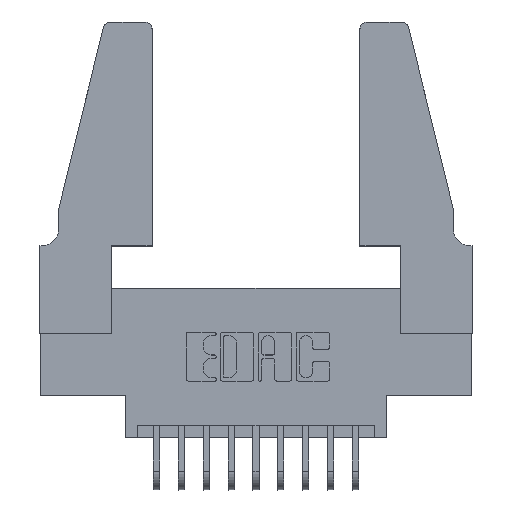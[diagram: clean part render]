
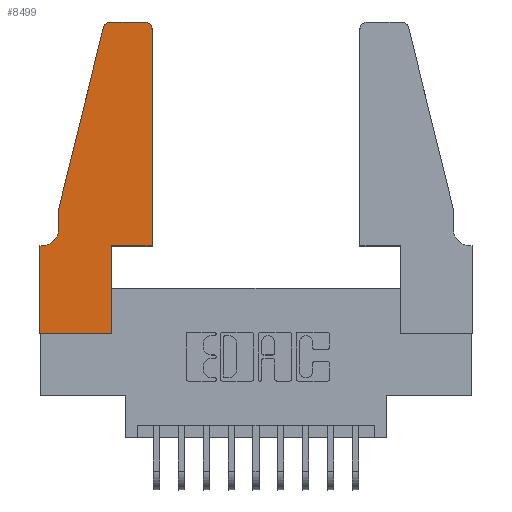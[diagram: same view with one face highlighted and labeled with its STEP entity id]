
A CAD part, top view. The second image highlights one B-rep face of the part: STEP entity #8499.
In plain terms, the highlighted planar face has unit normal (0, 0, 1).
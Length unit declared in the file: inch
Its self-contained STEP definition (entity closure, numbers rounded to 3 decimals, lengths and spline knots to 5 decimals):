
#67 = DIRECTION ( 'NONE',  ( 0., -1., 0. ) ) ;
#287 = ORIENTED_EDGE ( 'NONE', *, *, #6529, .T. ) ;
#686 = CARTESIAN_POINT ( 'NONE',  ( 0.0755, 0.35, 0.37 ) ) ;
#770 = DIRECTION ( 'NONE',  ( 1., 0., 0. ) ) ;
#864 = CIRCLE ( 'NONE', #10006, 0.03 ) ;
#869 = VERTEX_POINT ( 'NONE', #8610 ) ;
#890 = DIRECTION ( 'NONE',  ( -0.239, -0.971, 0. ) ) ;
#1489 = AXIS2_PLACEMENT_3D ( 'NONE', #1945, #5606, #13711 ) ;
#1795 = ORIENTED_EDGE ( 'NONE', *, *, #4038, .T. ) ;
#1843 = CARTESIAN_POINT ( 'NONE',  ( 0.0755, 0.42, 0.37 ) ) ;
#1945 = CARTESIAN_POINT ( 'NONE',  ( 0., 0.35, 0.37 ) ) ;
#1946 = VECTOR ( 'NONE', #9826, 39.37008 ) ;
#2008 = CARTESIAN_POINT ( 'NONE',  ( 0.4505, 0.35, 0.37 ) ) ;
#2247 = CARTESIAN_POINT ( 'NONE',  ( 0.284, 1.25, 0.37 ) ) ;
#2280 = VECTOR ( 'NONE', #3668, 39.37008 ) ;
#2497 = VECTOR ( 'NONE', #770, 39.37008 ) ;
#2616 = ORIENTED_EDGE ( 'NONE', *, *, #10988, .T. ) ;
#2724 = LINE ( 'NONE', #686, #8620 ) ;
#2897 = VERTEX_POINT ( 'NONE', #1843 ) ;
#3255 = CARTESIAN_POINT ( 'NONE',  ( 0.25487, 1.22718, 0.37 ) ) ;
#3314 = EDGE_CURVE ( 'NONE', #12942, #4967, #11859, .T. ) ;
#3324 = VERTEX_POINT ( 'NONE', #8568 ) ;
#3341 = DIRECTION ( 'NONE',  ( 1., 0., 0. ) ) ;
#3425 = ORIENTED_EDGE ( 'NONE', *, *, #8893, .T. ) ;
#3594 = VERTEX_POINT ( 'NONE', #8974 ) ;
#3668 = DIRECTION ( 'NONE',  ( 0., -1., 0. ) ) ;
#4038 = EDGE_CURVE ( 'NONE', #14106, #3324, #4765, .T. ) ;
#4055 = VECTOR ( 'NONE', #3341, 39.37008 ) ;
#4428 = CARTESIAN_POINT ( 'NONE',  ( 0.2605, 1.25, 0.37 ) ) ;
#4483 = FACE_OUTER_BOUND ( 'NONE', #13383, .T. ) ;
#4545 = CARTESIAN_POINT ( 'NONE',  ( 0., 0., 0.37 ) ) ;
#4765 = LINE ( 'NONE', #8649, #10584 ) ;
#4893 = VERTEX_POINT ( 'NONE', #3255 ) ;
#4896 = ORIENTED_EDGE ( 'NONE', *, *, #7492, .T. ) ;
#4967 = VERTEX_POINT ( 'NONE', #13349 ) ;
#5037 = DIRECTION ( 'NONE',  ( 0., 0., -1. ) ) ;
#5199 = LINE ( 'NONE', #14412, #1946 ) ;
#5317 = CARTESIAN_POINT ( 'NONE',  ( 0.284, 1.22, 0.37 ) ) ;
#5606 = DIRECTION ( 'NONE',  ( 0., 0., 1. ) ) ;
#6224 = DIRECTION ( 'NONE',  ( 0., 0., 1. ) ) ;
#6474 = DIRECTION ( 'NONE',  ( 1., 0., 0. ) ) ;
#6529 = EDGE_CURVE ( 'NONE', #2897, #3594, #13419, .T. ) ;
#6693 = LINE ( 'NONE', #4428, #9792 ) ;
#7492 = EDGE_CURVE ( 'NONE', #11521, #12942, #12670, .T. ) ;
#7604 = AXIS2_PLACEMENT_3D ( 'NONE', #11986, #5037, #13156 ) ;
#7667 = LINE ( 'NONE', #8152, #13856 ) ;
#7758 = CARTESIAN_POINT ( 'NONE',  ( 0.4505, 0.35, 0.37 ) ) ;
#7877 = LINE ( 'NONE', #9168, #4055 ) ;
#7952 = DIRECTION ( 'NONE',  ( 0., 1., 0. ) ) ;
#7994 = CARTESIAN_POINT ( 'NONE',  ( 0.4505, 1.22, 0.37 ) ) ;
#8015 = VERTEX_POINT ( 'NONE', #2247 ) ;
#8068 = ORIENTED_EDGE ( 'NONE', *, *, #10804, .T. ) ;
#8152 = CARTESIAN_POINT ( 'NONE',  ( 0.0755, 0.5, 0.37 ) ) ;
#8499 = ADVANCED_FACE ( 'NONE', ( #4483 ), #10242, .T. ) ;
#8568 = CARTESIAN_POINT ( 'NONE',  ( 0., 0., 0.37 ) ) ;
#8610 = CARTESIAN_POINT ( 'NONE',  ( 0.0755, 0.5, 0.37 ) ) ;
#8620 = VECTOR ( 'NONE', #10327, 39.37008 ) ;
#8649 = CARTESIAN_POINT ( 'NONE',  ( 0., 0., 0.37 ) ) ;
#8738 = ORIENTED_EDGE ( 'NONE', *, *, #10372, .T. ) ;
#8814 = CARTESIAN_POINT ( 'NONE',  ( 0.2865, 0., 0.37 ) ) ;
#8893 = EDGE_CURVE ( 'NONE', #8997, #9135, #5199, .T. ) ;
#8964 = LINE ( 'NONE', #9489, #2280 ) ;
#8974 = CARTESIAN_POINT ( 'NONE',  ( 0.0055, 0.35, 0.37 ) ) ;
#8997 = VERTEX_POINT ( 'NONE', #8814 ) ;
#9135 = VERTEX_POINT ( 'NONE', #14860 ) ;
#9168 = CARTESIAN_POINT ( 'NONE',  ( 0.4505, 0.35, 0.37 ) ) ;
#9227 = VECTOR ( 'NONE', #7952, 39.37008 ) ;
#9489 = CARTESIAN_POINT ( 'NONE',  ( 0.0755, 0.5, 0.37 ) ) ;
#9792 = VECTOR ( 'NONE', #10226, 39.37008 ) ;
#9802 = ORIENTED_EDGE ( 'NONE', *, *, #3314, .T. ) ;
#9826 = DIRECTION ( 'NONE',  ( 0., 1., 0. ) ) ;
#10006 = AXIS2_PLACEMENT_3D ( 'NONE', #5317, #13425, #6474 ) ;
#10226 = DIRECTION ( 'NONE',  ( -1., 0., 0. ) ) ;
#10242 = PLANE ( 'NONE',  #1489 ) ;
#10327 = DIRECTION ( 'NONE',  ( -1., 0., 0. ) ) ;
#10372 = EDGE_CURVE ( 'NONE', #3324, #8997, #15294, .T. ) ;
#10423 = EDGE_CURVE ( 'NONE', #4893, #869, #7667, .T. ) ;
#10447 = ORIENTED_EDGE ( 'NONE', *, *, #12411, .T. ) ;
#10584 = VECTOR ( 'NONE', #67, 39.37008 ) ;
#10804 = EDGE_CURVE ( 'NONE', #8015, #4893, #864, .T. ) ;
#10988 = EDGE_CURVE ( 'NONE', #9135, #11521, #7877, .T. ) ;
#11012 = CARTESIAN_POINT ( 'NONE',  ( 0., 0.35, 0.37 ) ) ;
#11252 = ORIENTED_EDGE ( 'NONE', *, *, #14768, .T. ) ;
#11521 = VERTEX_POINT ( 'NONE', #7758 ) ;
#11568 = EDGE_CURVE ( 'NONE', #3594, #14106, #2724, .T. ) ;
#11595 = ORIENTED_EDGE ( 'NONE', *, *, #11568, .T. ) ;
#11859 = CIRCLE ( 'NONE', #12042, 0.03 ) ;
#11986 = CARTESIAN_POINT ( 'NONE',  ( 0.0055, 0.42, 0.37 ) ) ;
#12042 = AXIS2_PLACEMENT_3D ( 'NONE', #13178, #6224, #14331 ) ;
#12411 = EDGE_CURVE ( 'NONE', #869, #2897, #8964, .T. ) ;
#12670 = LINE ( 'NONE', #2008, #9227 ) ;
#12942 = VERTEX_POINT ( 'NONE', #7994 ) ;
#13149 = ORIENTED_EDGE ( 'NONE', *, *, #10423, .T. ) ;
#13156 = DIRECTION ( 'NONE',  ( -1., 0., 0. ) ) ;
#13178 = CARTESIAN_POINT ( 'NONE',  ( 0.4205, 1.22, 0.37 ) ) ;
#13349 = CARTESIAN_POINT ( 'NONE',  ( 0.4205, 1.25, 0.37 ) ) ;
#13383 = EDGE_LOOP ( 'NONE', ( #11252, #8068, #13149, #10447, #287, #11595, #1795, #8738, #3425, #2616, #4896, #9802 ) ) ;
#13419 = CIRCLE ( 'NONE', #7604, 0.07 ) ;
#13425 = DIRECTION ( 'NONE',  ( 0., 0., 1. ) ) ;
#13711 = DIRECTION ( 'NONE',  ( 1., 0., 0. ) ) ;
#13856 = VECTOR ( 'NONE', #890, 39.37008 ) ;
#14106 = VERTEX_POINT ( 'NONE', #11012 ) ;
#14331 = DIRECTION ( 'NONE',  ( 1., 0., 0. ) ) ;
#14412 = CARTESIAN_POINT ( 'NONE',  ( 0.2865, 0.35, 0.37 ) ) ;
#14768 = EDGE_CURVE ( 'NONE', #4967, #8015, #6693, .T. ) ;
#14860 = CARTESIAN_POINT ( 'NONE',  ( 0.2865, 0.35, 0.37 ) ) ;
#15294 = LINE ( 'NONE', #4545, #2497 ) ;
